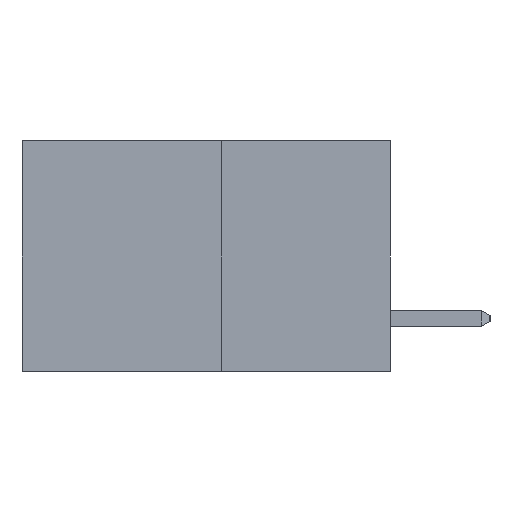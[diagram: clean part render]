
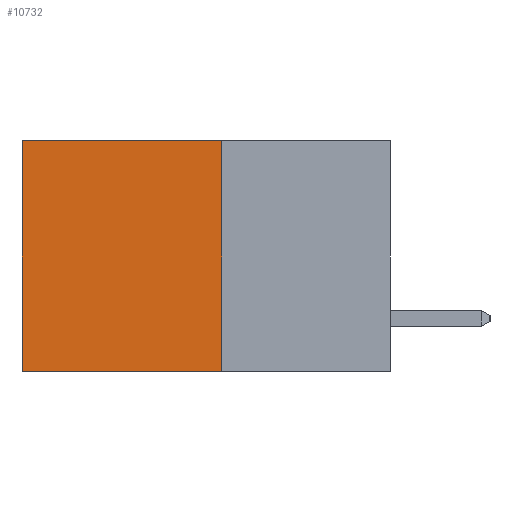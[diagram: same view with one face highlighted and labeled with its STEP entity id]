
A CAD part, left-side view. The second image highlights one B-rep face of the part: STEP entity #10732.
In plain terms, the highlighted planar face has unit normal (-1, 0, 0).
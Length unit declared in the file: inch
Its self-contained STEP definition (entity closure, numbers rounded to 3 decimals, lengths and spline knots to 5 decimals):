
#689 = CARTESIAN_POINT ( 'NONE',  ( 0.277, 0.27, -0.37 ) ) ;
#941 = VECTOR ( 'NONE', #19374, 39.37008 ) ;
#1960 = CARTESIAN_POINT ( 'NONE',  ( 0.277, 0.27, -0.37 ) ) ;
#3355 = PLANE ( 'NONE',  #7468 ) ;
#3922 = EDGE_CURVE ( 'NONE', #17487, #18670, #17247, .T. ) ;
#4081 = CARTESIAN_POINT ( 'NONE',  ( 0.277, 0.59, -0.37 ) ) ;
#4491 = VERTEX_POINT ( 'NONE', #11761 ) ;
#5602 = DIRECTION ( 'NONE',  ( 0., 0., -1. ) ) ;
#6932 = ORIENTED_EDGE ( 'NONE', *, *, #3922, .F. ) ;
#7468 = AXIS2_PLACEMENT_3D ( 'NONE', #18378, #18856, #5602 ) ;
#8627 = EDGE_LOOP ( 'NONE', ( #9029, #6932, #24740, #12308 ) ) ;
#8674 = DIRECTION ( 'NONE',  ( 0., 0., -1. ) ) ;
#9029 = ORIENTED_EDGE ( 'NONE', *, *, #26177, .T. ) ;
#9158 = VECTOR ( 'NONE', #8674, 39.37008 ) ;
#9832 = LINE ( 'NONE', #1960, #9158 ) ;
#10732 = ADVANCED_FACE ( 'NONE', ( #11601 ), #3355, .F. ) ;
#11016 = EDGE_CURVE ( 'NONE', #4491, #17487, #9832, .T. ) ;
#11601 = FACE_OUTER_BOUND ( 'NONE', #8627, .T. ) ;
#11761 = CARTESIAN_POINT ( 'NONE',  ( 0.277, 0.27, 0. ) ) ;
#11869 = DIRECTION ( 'NONE',  ( 0., 1., 0. ) ) ;
#12308 = ORIENTED_EDGE ( 'NONE', *, *, #27936, .T. ) ;
#12656 = LINE ( 'NONE', #4081, #18579 ) ;
#13278 = CARTESIAN_POINT ( 'NONE',  ( 0.277, 0.59, -0.37 ) ) ;
#16378 = LINE ( 'NONE', #27299, #27385 ) ;
#16618 = VERTEX_POINT ( 'NONE', #21861 ) ;
#17247 = LINE ( 'NONE', #19200, #941 ) ;
#17487 = VERTEX_POINT ( 'NONE', #689 ) ;
#18378 = CARTESIAN_POINT ( 'NONE',  ( 0.277, 0.27, -0.37 ) ) ;
#18579 = VECTOR ( 'NONE', #19563, 39.37008 ) ;
#18670 = VERTEX_POINT ( 'NONE', #13278 ) ;
#18856 = DIRECTION ( 'NONE',  ( 1., 0., 0. ) ) ;
#19200 = CARTESIAN_POINT ( 'NONE',  ( 0.277, 0.27, -0.37 ) ) ;
#19374 = DIRECTION ( 'NONE',  ( 0., 1., 0. ) ) ;
#19563 = DIRECTION ( 'NONE',  ( 0., 0., -1. ) ) ;
#21861 = CARTESIAN_POINT ( 'NONE',  ( 0.277, 0.59, 0. ) ) ;
#24740 = ORIENTED_EDGE ( 'NONE', *, *, #11016, .F. ) ;
#26177 = EDGE_CURVE ( 'NONE', #16618, #18670, #12656, .T. ) ;
#27299 = CARTESIAN_POINT ( 'NONE',  ( 0.277, 0.27, 0. ) ) ;
#27385 = VECTOR ( 'NONE', #11869, 39.37008 ) ;
#27936 = EDGE_CURVE ( 'NONE', #4491, #16618, #16378, .T. ) ;
